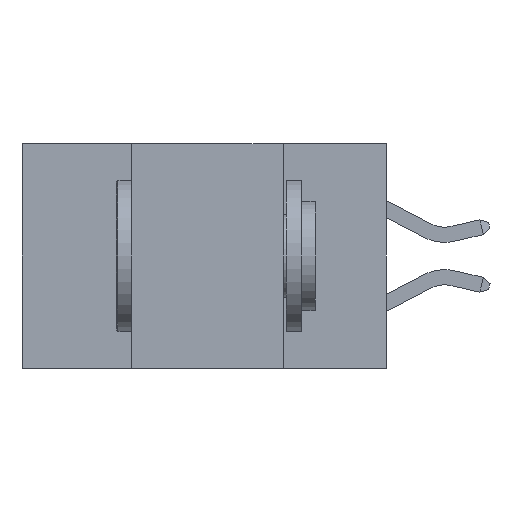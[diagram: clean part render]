
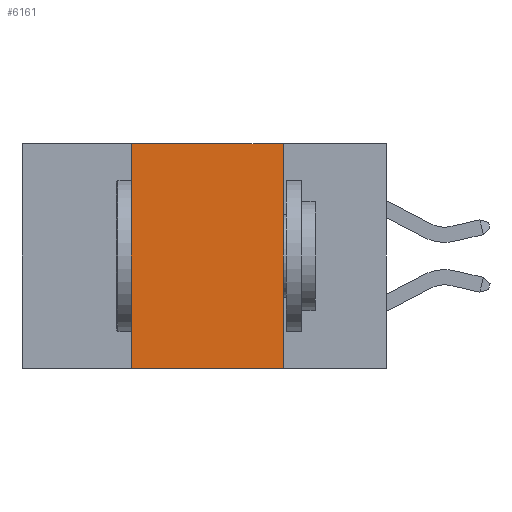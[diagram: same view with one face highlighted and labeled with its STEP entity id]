
A CAD part, left-side view. The second image highlights one B-rep face of the part: STEP entity #6161.
In plain terms, the highlighted planar face has unit normal (-1, 0, 0).
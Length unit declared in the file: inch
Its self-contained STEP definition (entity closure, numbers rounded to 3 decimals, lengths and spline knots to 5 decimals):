
#1163 = LINE ( 'NONE', #13160, #9614 ) ;
#1399 = DIRECTION ( 'NONE',  ( 1., 0., 0. ) ) ;
#1833 = EDGE_CURVE ( 'NONE', #5431, #5736, #1163, .T. ) ;
#1934 = EDGE_LOOP ( 'NONE', ( #10047, #10809, #10089, #11799 ) ) ;
#2646 = FACE_OUTER_BOUND ( 'NONE', #1934, .T. ) ;
#3658 = CARTESIAN_POINT ( 'NONE',  ( 0., 0.6, 0. ) ) ;
#4125 = EDGE_CURVE ( 'NONE', #5431, #11153, #19434, .T. ) ;
#4948 = CARTESIAN_POINT ( 'NONE',  ( 0., 0.42, -0.37 ) ) ;
#5397 = DIRECTION ( 'NONE',  ( 0., -1., 0. ) ) ;
#5405 = CARTESIAN_POINT ( 'NONE',  ( 0., 0.42, 0. ) ) ;
#5431 = VERTEX_POINT ( 'NONE', #4948 ) ;
#5630 = CARTESIAN_POINT ( 'NONE',  ( 0., 0.42, 0. ) ) ;
#5736 = VERTEX_POINT ( 'NONE', #6507 ) ;
#5834 = VERTEX_POINT ( 'NONE', #14279 ) ;
#6161 = ADVANCED_FACE ( 'NONE', ( #2646 ), #6469, .F. ) ;
#6462 = VECTOR ( 'NONE', #7817, 39.37008 ) ;
#6469 = PLANE ( 'NONE',  #14666 ) ;
#6507 = CARTESIAN_POINT ( 'NONE',  ( 0., 0.17, -0.37 ) ) ;
#7367 = LINE ( 'NONE', #18326, #11311 ) ;
#7520 = EDGE_CURVE ( 'NONE', #5834, #5736, #7367, .T. ) ;
#7817 = DIRECTION ( 'NONE',  ( 0., 0., 1. ) ) ;
#9608 = LINE ( 'NONE', #3658, #17742 ) ;
#9614 = VECTOR ( 'NONE', #16286, 39.37008 ) ;
#9819 = CARTESIAN_POINT ( 'NONE',  ( 0., 0.6, 0. ) ) ;
#10047 = ORIENTED_EDGE ( 'NONE', *, *, #7520, .F. ) ;
#10089 = ORIENTED_EDGE ( 'NONE', *, *, #4125, .F. ) ;
#10809 = ORIENTED_EDGE ( 'NONE', *, *, #11688, .F. ) ;
#11153 = VERTEX_POINT ( 'NONE', #5630 ) ;
#11311 = VECTOR ( 'NONE', #19922, 39.37008 ) ;
#11688 = EDGE_CURVE ( 'NONE', #11153, #5834, #9608, .T. ) ;
#11799 = ORIENTED_EDGE ( 'NONE', *, *, #1833, .T. ) ;
#13111 = DIRECTION ( 'NONE',  ( 0., 0., -1. ) ) ;
#13160 = CARTESIAN_POINT ( 'NONE',  ( 0., 0.6, -0.37 ) ) ;
#14279 = CARTESIAN_POINT ( 'NONE',  ( 0., 0.17, 0. ) ) ;
#14666 = AXIS2_PLACEMENT_3D ( 'NONE', #9819, #1399, #13111 ) ;
#16286 = DIRECTION ( 'NONE',  ( 0., -1., 0. ) ) ;
#17742 = VECTOR ( 'NONE', #5397, 39.37008 ) ;
#18326 = CARTESIAN_POINT ( 'NONE',  ( 0., 0.17, 0. ) ) ;
#19434 = LINE ( 'NONE', #5405, #6462 ) ;
#19922 = DIRECTION ( 'NONE',  ( 0., 0., -1. ) ) ;
